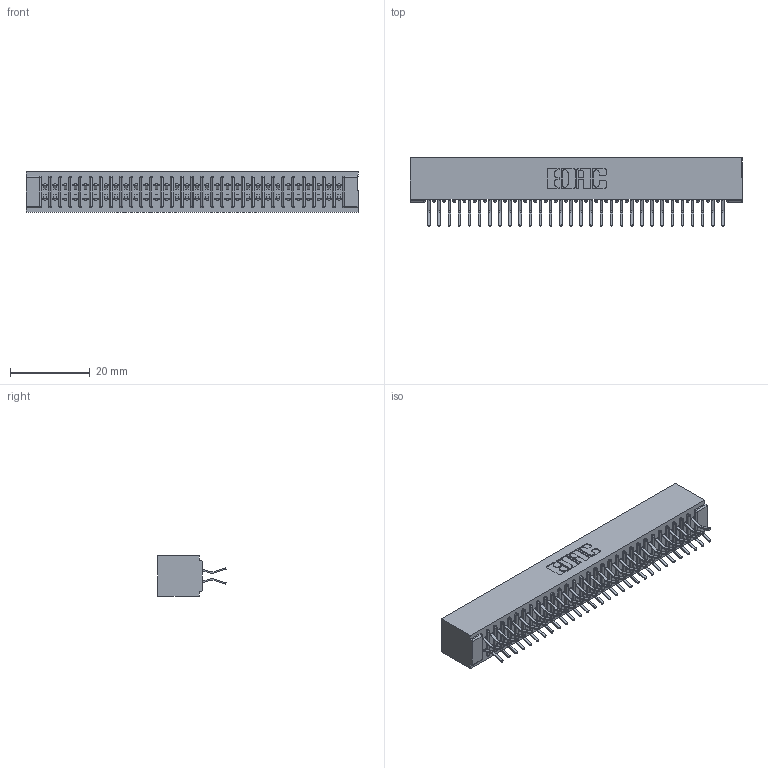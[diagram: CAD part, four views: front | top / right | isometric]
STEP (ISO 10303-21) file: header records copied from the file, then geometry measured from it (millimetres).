
FILE_DESCRIPTION (( 'STEP AP203' ), '1' );
FILE_NAME ('391-060-556-201.STEP', '2018-08-09T12:45:39', ( '' ), ( '' ), 'SwSTEP 2.0', 'SolidWorks 2016', '' );
FILE_SCHEMA (( 'CONFIG_CONTROL_DESIGN' ));
Length unit declared in the file: inch
Products named in the file (3): 341 Part_No Mounting Lugs; 341-292-001_341-292-156; 391-060-556-201
Assembly tree (61 placements, depth 2):
  391-060-556-201
    341 Part_No Mounting Lugs
    341-292-001_341-292-156  x60
Bounding box: 83.19 x 17.07 x 10.16 mm (x, y, z)
Volume: 6387.2 mm3; surface area: 11764.9 mm2
Topology: 61 solids, 61 shells, 4308 faces, 12502 edges, 8110 vertices
Faces by surface type: plane 2464, cylinder 1724, sphere 62, torus 58
Entity records: 37767 total; most frequent: CARTESIAN_POINT 6278, ORIENTED_EDGE 6236, DIRECTION 6104, EDGE_CURVE 3118, VECTOR 2504, LINE 2504, VERTEX_POINT 1974, AXIS2_PLACEMENT_3D 1800
